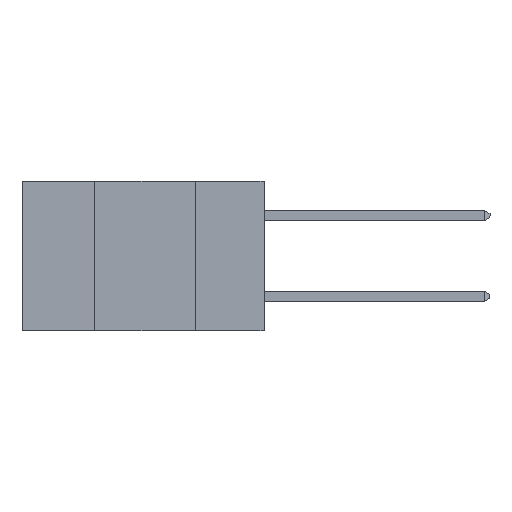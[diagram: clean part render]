
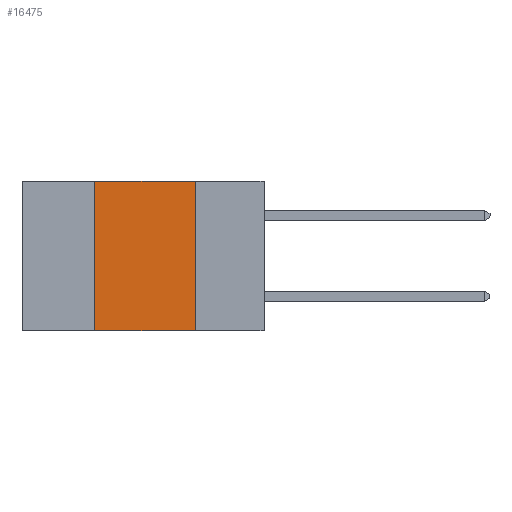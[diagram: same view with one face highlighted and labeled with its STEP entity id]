
A CAD part, left-side view. The second image highlights one B-rep face of the part: STEP entity #16475.
In plain terms, the highlighted planar face has unit normal (-1, 0, 0).
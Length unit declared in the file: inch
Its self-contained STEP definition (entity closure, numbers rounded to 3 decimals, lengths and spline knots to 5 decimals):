
#1751 = LINE ( 'NONE', #16718, #11092 ) ;
#1776 = PLANE ( 'NONE',  #9451 ) ;
#1855 = DIRECTION ( 'NONE',  ( 1., 0., 0. ) ) ;
#2528 = ORIENTED_EDGE ( 'NONE', *, *, #11647, .F. ) ;
#3569 = CARTESIAN_POINT ( 'NONE',  ( 0., 0.42, 0. ) ) ;
#4316 = CARTESIAN_POINT ( 'NONE',  ( 0., 0.42, -0.37 ) ) ;
#4463 = EDGE_CURVE ( 'NONE', #13269, #10878, #17622, .T. ) ;
#4614 = CARTESIAN_POINT ( 'NONE',  ( 0., 0.6, -0.37 ) ) ;
#5114 = EDGE_CURVE ( 'NONE', #13898, #10878, #22574, .T. ) ;
#5270 = EDGE_CURVE ( 'NONE', #13269, #19937, #10155, .T. ) ;
#6416 = DIRECTION ( 'NONE',  ( 0., 0., 1. ) ) ;
#6979 = ORIENTED_EDGE ( 'NONE', *, *, #5114, .F. ) ;
#8149 = ORIENTED_EDGE ( 'NONE', *, *, #5270, .F. ) ;
#9335 = CARTESIAN_POINT ( 'NONE',  ( 0., 0.6, 0. ) ) ;
#9451 = AXIS2_PLACEMENT_3D ( 'NONE', #9335, #1855, #14846 ) ;
#9585 = VECTOR ( 'NONE', #6416, 39.37008 ) ;
#10155 = LINE ( 'NONE', #3569, #9585 ) ;
#10878 = VERTEX_POINT ( 'NONE', #12833 ) ;
#11092 = VECTOR ( 'NONE', #18543, 39.37008 ) ;
#11647 = EDGE_CURVE ( 'NONE', #19937, #13898, #1751, .T. ) ;
#12179 = VECTOR ( 'NONE', #16287, 39.37008 ) ;
#12833 = CARTESIAN_POINT ( 'NONE',  ( 0., 0.17, -0.37 ) ) ;
#13269 = VERTEX_POINT ( 'NONE', #4316 ) ;
#13706 = CARTESIAN_POINT ( 'NONE',  ( 0., 0.17, 0. ) ) ;
#13898 = VERTEX_POINT ( 'NONE', #18850 ) ;
#14846 = DIRECTION ( 'NONE',  ( 0., 0., -1. ) ) ;
#16287 = DIRECTION ( 'NONE',  ( 0., -1., 0. ) ) ;
#16475 = ADVANCED_FACE ( 'NONE', ( #22270 ), #1776, .F. ) ;
#16718 = CARTESIAN_POINT ( 'NONE',  ( 0., 0.6, 0. ) ) ;
#17391 = DIRECTION ( 'NONE',  ( 0., 0., -1. ) ) ;
#17622 = LINE ( 'NONE', #4614, #12179 ) ;
#17863 = ORIENTED_EDGE ( 'NONE', *, *, #4463, .T. ) ;
#18444 = VECTOR ( 'NONE', #17391, 39.37008 ) ;
#18543 = DIRECTION ( 'NONE',  ( 0., -1., 0. ) ) ;
#18850 = CARTESIAN_POINT ( 'NONE',  ( 0., 0.17, 0. ) ) ;
#19656 = EDGE_LOOP ( 'NONE', ( #6979, #2528, #8149, #17863 ) ) ;
#19937 = VERTEX_POINT ( 'NONE', #21162 ) ;
#21162 = CARTESIAN_POINT ( 'NONE',  ( 0., 0.42, 0. ) ) ;
#22270 = FACE_OUTER_BOUND ( 'NONE', #19656, .T. ) ;
#22574 = LINE ( 'NONE', #13706, #18444 ) ;
